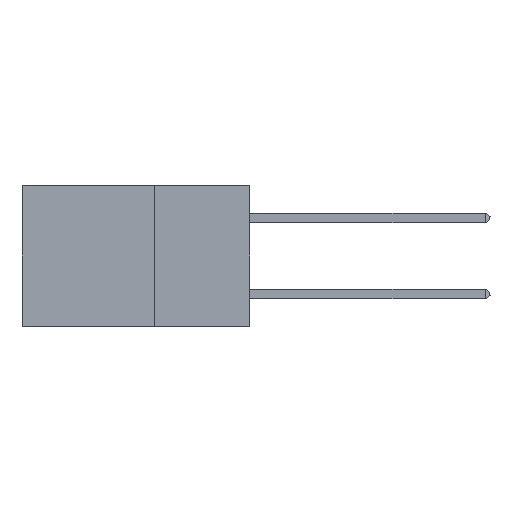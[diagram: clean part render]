
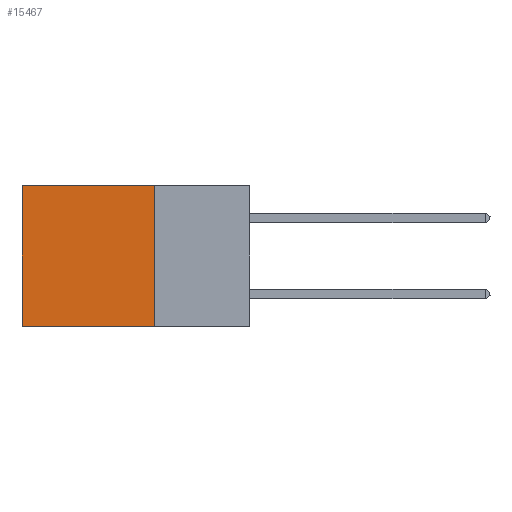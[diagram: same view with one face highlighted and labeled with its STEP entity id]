
A CAD part, left-side view. The second image highlights one B-rep face of the part: STEP entity #15467.
In plain terms, the highlighted planar face has unit normal (-1, 0, 0).
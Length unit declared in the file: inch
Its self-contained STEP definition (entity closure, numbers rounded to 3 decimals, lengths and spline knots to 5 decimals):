
#188 = ORIENTED_EDGE ( 'NONE', *, *, #8476, .T. ) ;
#1876 = VERTEX_POINT ( 'NONE', #4878 ) ;
#3312 = PLANE ( 'NONE',  #11045 ) ;
#3725 = ORIENTED_EDGE ( 'NONE', *, *, #5600, .F. ) ;
#4878 = CARTESIAN_POINT ( 'NONE',  ( 0.2875, 0.25, -0.37 ) ) ;
#5600 = EDGE_CURVE ( 'NONE', #14328, #1876, #16518, .T. ) ;
#5738 = CARTESIAN_POINT ( 'NONE',  ( 0.2875, 0.6, 0. ) ) ;
#6351 = CARTESIAN_POINT ( 'NONE',  ( 0.2875, 0.25, 0. ) ) ;
#6495 = DIRECTION ( 'NONE',  ( 0., 0., -1. ) ) ;
#7158 = CARTESIAN_POINT ( 'NONE',  ( 0.2875, 0.25, 0. ) ) ;
#7213 = LINE ( 'NONE', #29618, #10893 ) ;
#7293 = VECTOR ( 'NONE', #32625, 39.37008 ) ;
#8104 = VERTEX_POINT ( 'NONE', #16546 ) ;
#8407 = CARTESIAN_POINT ( 'NONE',  ( 0.2875, 0.25, 0. ) ) ;
#8476 = EDGE_CURVE ( 'NONE', #14328, #16196, #32528, .T. ) ;
#8525 = DIRECTION ( 'NONE',  ( 1., 0., 0. ) ) ;
#8578 = EDGE_CURVE ( 'NONE', #1876, #8104, #12647, .T. ) ;
#10210 = ORIENTED_EDGE ( 'NONE', *, *, #8578, .F. ) ;
#10893 = VECTOR ( 'NONE', #32280, 39.37008 ) ;
#11045 = AXIS2_PLACEMENT_3D ( 'NONE', #8407, #8525, #11285 ) ;
#11285 = DIRECTION ( 'NONE',  ( 0., 0., -1. ) ) ;
#11441 = CARTESIAN_POINT ( 'NONE',  ( 0.2875, 0.25, -0.37 ) ) ;
#12647 = LINE ( 'NONE', #11441, #7293 ) ;
#13156 = ORIENTED_EDGE ( 'NONE', *, *, #21692, .T. ) ;
#14328 = VERTEX_POINT ( 'NONE', #6351 ) ;
#15467 = ADVANCED_FACE ( 'NONE', ( #17411 ), #3312, .F. ) ;
#15560 = VECTOR ( 'NONE', #21623, 39.37008 ) ;
#15965 = CARTESIAN_POINT ( 'NONE',  ( 0.2875, 0.25, 0. ) ) ;
#16120 = VECTOR ( 'NONE', #6495, 39.37008 ) ;
#16196 = VERTEX_POINT ( 'NONE', #5738 ) ;
#16518 = LINE ( 'NONE', #7158, #16120 ) ;
#16546 = CARTESIAN_POINT ( 'NONE',  ( 0.2875, 0.6, -0.37 ) ) ;
#17411 = FACE_OUTER_BOUND ( 'NONE', #17756, .T. ) ;
#17756 = EDGE_LOOP ( 'NONE', ( #13156, #10210, #3725, #188 ) ) ;
#21623 = DIRECTION ( 'NONE',  ( 0., 1., 0. ) ) ;
#21692 = EDGE_CURVE ( 'NONE', #16196, #8104, #7213, .T. ) ;
#29618 = CARTESIAN_POINT ( 'NONE',  ( 0.2875, 0.6, 0. ) ) ;
#32280 = DIRECTION ( 'NONE',  ( 0., 0., -1. ) ) ;
#32528 = LINE ( 'NONE', #15965, #15560 ) ;
#32625 = DIRECTION ( 'NONE',  ( 0., 1., 0. ) ) ;
